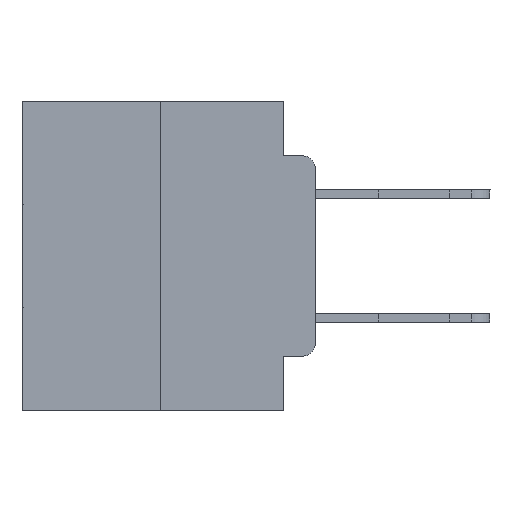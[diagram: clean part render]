
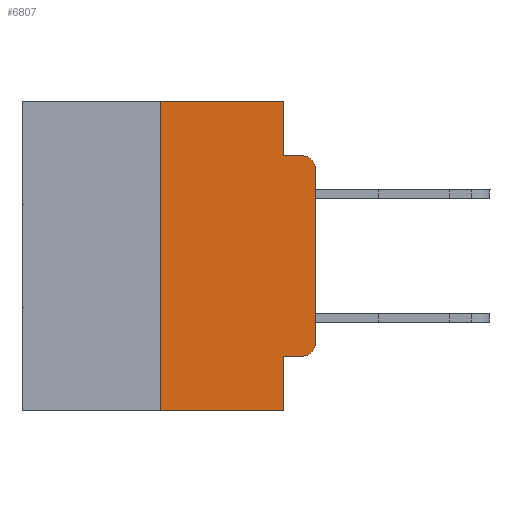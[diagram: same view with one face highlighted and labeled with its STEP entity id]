
A CAD part, left-side view. The second image highlights one B-rep face of the part: STEP entity #6807.
In plain terms, the highlighted planar face has unit normal (-1, 0, 0).
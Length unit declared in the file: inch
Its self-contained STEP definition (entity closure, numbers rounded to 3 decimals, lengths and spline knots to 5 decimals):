
#728 = DIRECTION ( 'NONE',  ( 0., 0., 1. ) ) ;
#753 = LINE ( 'NONE', #2563, #19006 ) ;
#969 = CARTESIAN_POINT ( 'NONE',  ( 0., 0.051, -0.5 ) ) ;
#1428 = CARTESIAN_POINT ( 'NONE',  ( 0., 0., -0.3915 ) ) ;
#2080 = DIRECTION ( 'NONE',  ( 0., 0., 1. ) ) ;
#2162 = CARTESIAN_POINT ( 'NONE',  ( 0., 0.051, -0.4115 ) ) ;
#2446 = VECTOR ( 'NONE', #728, 39.37008 ) ;
#2540 = ORIENTED_EDGE ( 'NONE', *, *, #18620, .T. ) ;
#2563 = CARTESIAN_POINT ( 'NONE',  ( 0., 0.051, 0. ) ) ;
#3027 = FACE_OUTER_BOUND ( 'NONE', #20302, .T. ) ;
#3229 = ORIENTED_EDGE ( 'NONE', *, *, #18851, .F. ) ;
#3520 = VECTOR ( 'NONE', #2080, 39.37008 ) ;
#3857 = EDGE_CURVE ( 'NONE', #17151, #8554, #753, .T. ) ;
#4089 = VECTOR ( 'NONE', #19434, 39.37008 ) ;
#4466 = CARTESIAN_POINT ( 'NONE',  ( 0., 0.02, -0.0885 ) ) ;
#5837 = EDGE_CURVE ( 'NONE', #15356, #7818, #11388, .T. ) ;
#6063 = EDGE_CURVE ( 'NONE', #9544, #7613, #22596, .T. ) ;
#6239 = CARTESIAN_POINT ( 'NONE',  ( 0., 0.051, 0. ) ) ;
#6359 = LINE ( 'NONE', #21596, #3520 ) ;
#6783 = AXIS2_PLACEMENT_3D ( 'NONE', #22880, #8052, #7914 ) ;
#6807 = ADVANCED_FACE ( 'NONE', ( #3027 ), #11581, .F. ) ;
#7561 = CARTESIAN_POINT ( 'NONE',  ( 0., 0.473, 0. ) ) ;
#7597 = VERTEX_POINT ( 'NONE', #22300 ) ;
#7613 = VERTEX_POINT ( 'NONE', #969 ) ;
#7818 = VERTEX_POINT ( 'NONE', #25075 ) ;
#7914 = DIRECTION ( 'NONE',  ( 0., 0., -1. ) ) ;
#8052 = DIRECTION ( 'NONE',  ( -1., 0., 0. ) ) ;
#8110 = VERTEX_POINT ( 'NONE', #17534 ) ;
#8554 = VERTEX_POINT ( 'NONE', #11934 ) ;
#9157 = VECTOR ( 'NONE', #12046, 39.37008 ) ;
#9544 = VERTEX_POINT ( 'NONE', #15071 ) ;
#9693 = LINE ( 'NONE', #22328, #26707 ) ;
#9840 = DIRECTION ( 'NONE',  ( 0., -1., 0. ) ) ;
#9875 = AXIS2_PLACEMENT_3D ( 'NONE', #22056, #17590, #15800 ) ;
#10153 = LINE ( 'NONE', #11817, #20030 ) ;
#10566 = ORIENTED_EDGE ( 'NONE', *, *, #21645, .F. ) ;
#10645 = DIRECTION ( 'NONE',  ( 0., -1., 0. ) ) ;
#10844 = ORIENTED_EDGE ( 'NONE', *, *, #20068, .T. ) ;
#11388 = LINE ( 'NONE', #26614, #2446 ) ;
#11581 = PLANE ( 'NONE',  #18535 ) ;
#11817 = CARTESIAN_POINT ( 'NONE',  ( 0., 0.473, 0. ) ) ;
#11934 = CARTESIAN_POINT ( 'NONE',  ( 0., 0.051, -0.0885 ) ) ;
#12046 = DIRECTION ( 'NONE',  ( 0., 0., -1. ) ) ;
#12138 = CARTESIAN_POINT ( 'NONE',  ( 0., 0.02, -0.4115 ) ) ;
#12229 = DIRECTION ( 'NONE',  ( 0., -1., 0. ) ) ;
#13957 = ORIENTED_EDGE ( 'NONE', *, *, #21626, .T. ) ;
#14180 = DIRECTION ( 'NONE',  ( 1., 0., 0. ) ) ;
#14579 = ORIENTED_EDGE ( 'NONE', *, *, #18342, .F. ) ;
#14982 = VERTEX_POINT ( 'NONE', #4466 ) ;
#15071 = CARTESIAN_POINT ( 'NONE',  ( 0., 0.051, -0.4115 ) ) ;
#15356 = VERTEX_POINT ( 'NONE', #1428 ) ;
#15709 = ORIENTED_EDGE ( 'NONE', *, *, #5837, .T. ) ;
#15800 = DIRECTION ( 'NONE',  ( 0., 0., -1. ) ) ;
#17151 = VERTEX_POINT ( 'NONE', #25116 ) ;
#17534 = CARTESIAN_POINT ( 'NONE',  ( 0., 0.25, -0.5 ) ) ;
#17590 = DIRECTION ( 'NONE',  ( -1., 0., 0. ) ) ;
#17610 = DIRECTION ( 'NONE',  ( 0., 0., -1. ) ) ;
#18342 = EDGE_CURVE ( 'NONE', #7597, #17151, #10153, .T. ) ;
#18535 = AXIS2_PLACEMENT_3D ( 'NONE', #7561, #14180, #22390 ) ;
#18620 = EDGE_CURVE ( 'NONE', #7818, #14982, #20883, .T. ) ;
#18851 = EDGE_CURVE ( 'NONE', #8554, #14982, #9693, .T. ) ;
#19006 = VECTOR ( 'NONE', #17610, 39.37008 ) ;
#19298 = EDGE_CURVE ( 'NONE', #9544, #25988, #21557, .T. ) ;
#19434 = DIRECTION ( 'NONE',  ( 0., -1., 0. ) ) ;
#19807 = ORIENTED_EDGE ( 'NONE', *, *, #6063, .F. ) ;
#20030 = VECTOR ( 'NONE', #12229, 39.37008 ) ;
#20068 = EDGE_CURVE ( 'NONE', #25988, #15356, #24958, .T. ) ;
#20302 = EDGE_LOOP ( 'NONE', ( #15709, #2540, #3229, #24896, #14579, #10566, #13957, #19807, #26120, #10844 ) ) ;
#20883 = CIRCLE ( 'NONE', #9875, 0.02 ) ;
#21323 = CARTESIAN_POINT ( 'NONE',  ( 0., 0.473, -0.5 ) ) ;
#21557 = LINE ( 'NONE', #2162, #4089 ) ;
#21596 = CARTESIAN_POINT ( 'NONE',  ( 0., 0.25, 0. ) ) ;
#21626 = EDGE_CURVE ( 'NONE', #8110, #7613, #25214, .T. ) ;
#21645 = EDGE_CURVE ( 'NONE', #8110, #7597, #6359, .T. ) ;
#21647 = VECTOR ( 'NONE', #10645, 39.37008 ) ;
#22056 = CARTESIAN_POINT ( 'NONE',  ( 0., 0.02, -0.1085 ) ) ;
#22300 = CARTESIAN_POINT ( 'NONE',  ( 0., 0.25, 0. ) ) ;
#22328 = CARTESIAN_POINT ( 'NONE',  ( 0., 0.051, -0.0885 ) ) ;
#22390 = DIRECTION ( 'NONE',  ( 0., 0., -1. ) ) ;
#22596 = LINE ( 'NONE', #6239, #9157 ) ;
#22880 = CARTESIAN_POINT ( 'NONE',  ( 0., 0.02, -0.3915 ) ) ;
#24896 = ORIENTED_EDGE ( 'NONE', *, *, #3857, .F. ) ;
#24958 = CIRCLE ( 'NONE', #6783, 0.02 ) ;
#25075 = CARTESIAN_POINT ( 'NONE',  ( 0., 0., -0.1085 ) ) ;
#25116 = CARTESIAN_POINT ( 'NONE',  ( 0., 0.051, 0. ) ) ;
#25214 = LINE ( 'NONE', #21323, #21647 ) ;
#25988 = VERTEX_POINT ( 'NONE', #12138 ) ;
#26120 = ORIENTED_EDGE ( 'NONE', *, *, #19298, .T. ) ;
#26614 = CARTESIAN_POINT ( 'NONE',  ( 0., 0., 0. ) ) ;
#26707 = VECTOR ( 'NONE', #9840, 39.37008 ) ;
